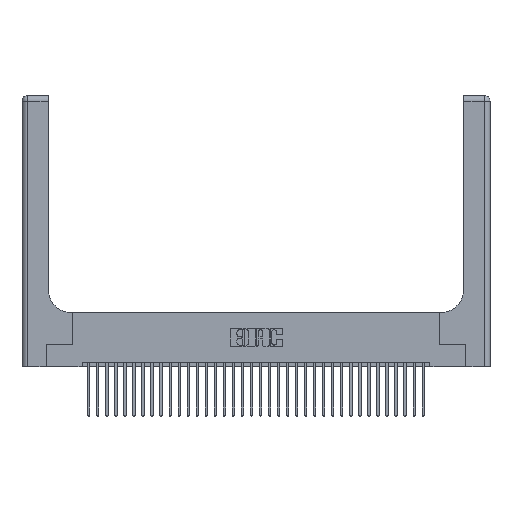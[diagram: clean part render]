
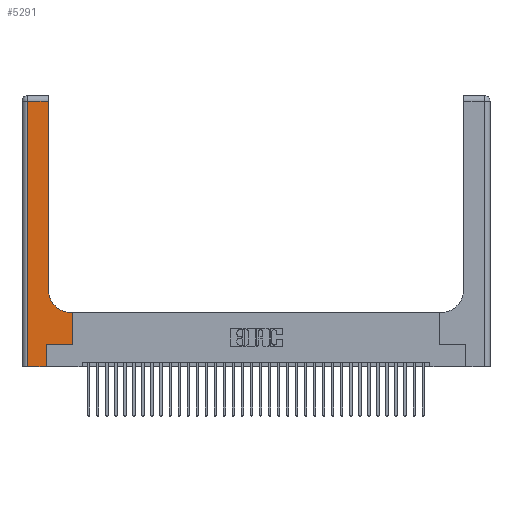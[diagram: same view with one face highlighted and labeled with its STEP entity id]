
A CAD part, top view. The second image highlights one B-rep face of the part: STEP entity #5291.
In plain terms, the highlighted planar face has unit normal (0, 0, 1).
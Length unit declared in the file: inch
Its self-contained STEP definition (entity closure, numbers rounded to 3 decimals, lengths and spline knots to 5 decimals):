
#211 = EDGE_CURVE ( 'NONE', #30304, #12991, #31422, .T. ) ;
#776 = DIRECTION ( 'NONE',  ( 0., 1., 0. ) ) ;
#1176 = LINE ( 'NONE', #29011, #14525 ) ;
#1249 = VERTEX_POINT ( 'NONE', #15463 ) ;
#1390 = DIRECTION ( 'NONE',  ( 1., 0., 0. ) ) ;
#1505 = LINE ( 'NONE', #30328, #13557 ) ;
#2091 = LINE ( 'NONE', #6469, #2490 ) ;
#2413 = DIRECTION ( 'NONE',  ( 0., 0., -1. ) ) ;
#2490 = VECTOR ( 'NONE', #30997, 39.37008 ) ;
#3306 = VERTEX_POINT ( 'NONE', #30082 ) ;
#3546 = EDGE_CURVE ( 'NONE', #3306, #1249, #1505, .T. ) ;
#4106 = CARTESIAN_POINT ( 'NONE',  ( 0.2915, 2.94, 0.37 ) ) ;
#5291 = ADVANCED_FACE ( 'NONE', ( #29595 ), #32101, .F. ) ;
#5550 = VECTOR ( 'NONE', #12105, 39.37008 ) ;
#5923 = CARTESIAN_POINT ( 'NONE',  ( 0.2915, 3., 0.37 ) ) ;
#6469 = CARTESIAN_POINT ( 'NONE',  ( 0.06, 3., 0.37 ) ) ;
#7352 = DIRECTION ( 'NONE',  ( -1., 0., 0. ) ) ;
#7777 = EDGE_CURVE ( 'NONE', #1249, #28680, #14774, .T. ) ;
#8147 = LINE ( 'NONE', #31115, #5550 ) ;
#8305 = EDGE_CURVE ( 'NONE', #21372, #26715, #24626, .T. ) ;
#9096 = DIRECTION ( 'NONE',  ( 0., 1., 0. ) ) ;
#10039 = VECTOR ( 'NONE', #20663, 39.37008 ) ;
#11121 = EDGE_CURVE ( 'NONE', #28680, #19208, #1176, .T. ) ;
#11210 = CARTESIAN_POINT ( 'NONE',  ( 0.269, 0.25, 0.37 ) ) ;
#12050 = AXIS2_PLACEMENT_3D ( 'NONE', #18556, #24568, #21462 ) ;
#12105 = DIRECTION ( 'NONE',  ( -1., 0., 0. ) ) ;
#12173 = VECTOR ( 'NONE', #9096, 39.37008 ) ;
#12991 = VERTEX_POINT ( 'NONE', #29801 ) ;
#13071 = LINE ( 'NONE', #17626, #10039 ) ;
#13557 = VECTOR ( 'NONE', #22667, 39.37008 ) ;
#13729 = ORIENTED_EDGE ( 'NONE', *, *, #7777, .T. ) ;
#13895 = CARTESIAN_POINT ( 'NONE',  ( 0.06, 2.94, 0.37 ) ) ;
#13956 = AXIS2_PLACEMENT_3D ( 'NONE', #32581, #2413, #7352 ) ;
#14525 = VECTOR ( 'NONE', #1390, 39.37008 ) ;
#14726 = ORIENTED_EDGE ( 'NONE', *, *, #25412, .T. ) ;
#14774 = LINE ( 'NONE', #30862, #12173 ) ;
#15432 = CARTESIAN_POINT ( 'NONE',  ( 0.5585, 0.6, 0.37 ) ) ;
#15463 = CARTESIAN_POINT ( 'NONE',  ( 0.269, 0., 0.37 ) ) ;
#16037 = EDGE_CURVE ( 'NONE', #26715, #21149, #8147, .T. ) ;
#16251 = ORIENTED_EDGE ( 'NONE', *, *, #11121, .T. ) ;
#17626 = CARTESIAN_POINT ( 'NONE',  ( 0.5585, 0.25, 0.37 ) ) ;
#18556 = CARTESIAN_POINT ( 'NONE',  ( 0.5415, 0.85, 0.37 ) ) ;
#19056 = ORIENTED_EDGE ( 'NONE', *, *, #16037, .T. ) ;
#19170 = ORIENTED_EDGE ( 'NONE', *, *, #20116, .T. ) ;
#19208 = VERTEX_POINT ( 'NONE', #24320 ) ;
#20116 = EDGE_CURVE ( 'NONE', #21149, #3306, #2091, .T. ) ;
#20663 = DIRECTION ( 'NONE',  ( 0., 1., 0. ) ) ;
#21149 = VERTEX_POINT ( 'NONE', #13895 ) ;
#21372 = VERTEX_POINT ( 'NONE', #23225 ) ;
#21462 = DIRECTION ( 'NONE',  ( 1., 0., 0. ) ) ;
#22379 = ORIENTED_EDGE ( 'NONE', *, *, #3546, .T. ) ;
#22667 = DIRECTION ( 'NONE',  ( 1., 0., 0. ) ) ;
#23225 = CARTESIAN_POINT ( 'NONE',  ( 0.2915, 0.85, 0.37 ) ) ;
#24288 = CIRCLE ( 'NONE', #12050, 0.25 ) ;
#24320 = CARTESIAN_POINT ( 'NONE',  ( 0.5585, 0.25, 0.37 ) ) ;
#24568 = DIRECTION ( 'NONE',  ( 0., 0., -1. ) ) ;
#24626 = LINE ( 'NONE', #5923, #28071 ) ;
#25412 = EDGE_CURVE ( 'NONE', #19208, #30304, #13071, .T. ) ;
#26715 = VERTEX_POINT ( 'NONE', #4106 ) ;
#28071 = VECTOR ( 'NONE', #776, 39.37008 ) ;
#28467 = ORIENTED_EDGE ( 'NONE', *, *, #8305, .T. ) ;
#28680 = VERTEX_POINT ( 'NONE', #11210 ) ;
#28847 = EDGE_LOOP ( 'NONE', ( #28467, #19056, #19170, #22379, #13729, #16251, #14726, #31919, #32742 ) ) ;
#29011 = CARTESIAN_POINT ( 'NONE',  ( 0.269, 0.25, 0.37 ) ) ;
#29595 = FACE_OUTER_BOUND ( 'NONE', #28847, .T. ) ;
#29702 = VECTOR ( 'NONE', #35087, 39.37008 ) ;
#29801 = CARTESIAN_POINT ( 'NONE',  ( 0.5415, 0.6, 0.37 ) ) ;
#30082 = CARTESIAN_POINT ( 'NONE',  ( 0.06, 0., 0.37 ) ) ;
#30304 = VERTEX_POINT ( 'NONE', #15432 ) ;
#30328 = CARTESIAN_POINT ( 'NONE',  ( 0., 0., 0.37 ) ) ;
#30862 = CARTESIAN_POINT ( 'NONE',  ( 0.269, 0., 0.37 ) ) ;
#30997 = DIRECTION ( 'NONE',  ( 0., -1., 0. ) ) ;
#31115 = CARTESIAN_POINT ( 'NONE',  ( 0., 2.94, 0.37 ) ) ;
#31422 = LINE ( 'NONE', #35324, #29702 ) ;
#31919 = ORIENTED_EDGE ( 'NONE', *, *, #211, .T. ) ;
#32101 = PLANE ( 'NONE',  #13956 ) ;
#32581 = CARTESIAN_POINT ( 'NONE',  ( 0., 3., 0.37 ) ) ;
#32742 = ORIENTED_EDGE ( 'NONE', *, *, #33735, .T. ) ;
#33735 = EDGE_CURVE ( 'NONE', #12991, #21372, #24288, .T. ) ;
#35087 = DIRECTION ( 'NONE',  ( -1., 0., 0. ) ) ;
#35324 = CARTESIAN_POINT ( 'NONE',  ( 0.2915, 0.6, 0.37 ) ) ;
